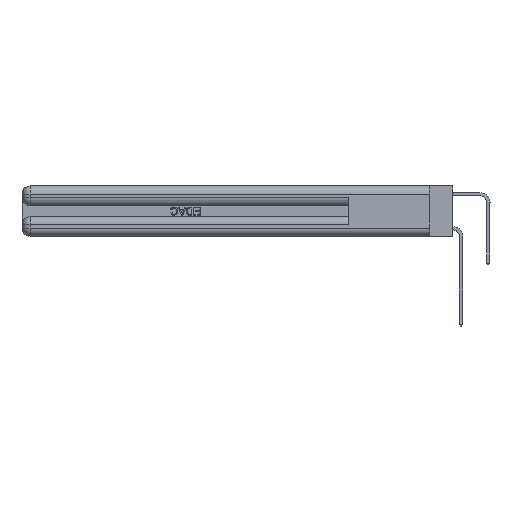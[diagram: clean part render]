
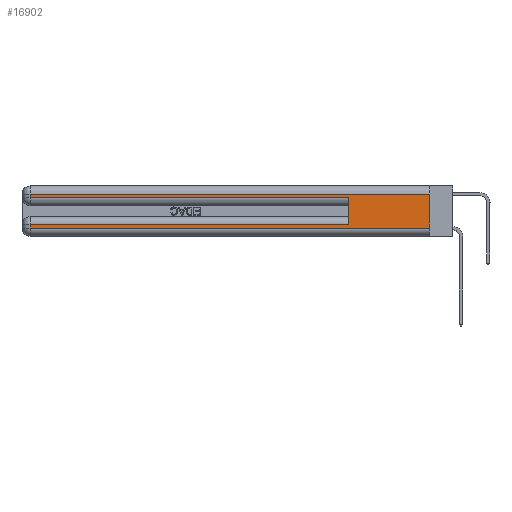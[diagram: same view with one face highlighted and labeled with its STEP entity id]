
A CAD part, left-side view. The second image highlights one B-rep face of the part: STEP entity #16902.
In plain terms, the highlighted planar face has unit normal (-1, 0, 0).
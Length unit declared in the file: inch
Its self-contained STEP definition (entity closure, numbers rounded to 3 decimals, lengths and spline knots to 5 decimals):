
#387 = ORIENTED_EDGE ( 'NONE', *, *, #13676, .T. ) ;
#787 = ORIENTED_EDGE ( 'NONE', *, *, #15017, .F. ) ;
#1704 = ORIENTED_EDGE ( 'NONE', *, *, #35412, .T. ) ;
#2054 = VERTEX_POINT ( 'NONE', #36527 ) ;
#2170 = LINE ( 'NONE', #22982, #8483 ) ;
#2703 = VERTEX_POINT ( 'NONE', #21536 ) ;
#3067 = VECTOR ( 'NONE', #14530, 39.37008 ) ;
#3115 = ORIENTED_EDGE ( 'NONE', *, *, #11278, .T. ) ;
#4183 = CARTESIAN_POINT ( 'NONE',  ( 0., 0., 0.31 ) ) ;
#4796 = FACE_OUTER_BOUND ( 'NONE', #35526, .T. ) ;
#5351 = DIRECTION ( 'NONE',  ( 0., -1., 0. ) ) ;
#6927 = CARTESIAN_POINT ( 'NONE',  ( 0., 0., 0.31 ) ) ;
#8483 = VECTOR ( 'NONE', #12206, 39.37008 ) ;
#8495 = VERTEX_POINT ( 'NONE', #32605 ) ;
#8623 = DIRECTION ( 'NONE',  ( 0., 0., -1. ) ) ;
#8759 = VECTOR ( 'NONE', #23881, 39.37008 ) ;
#9619 = VECTOR ( 'NONE', #36544, 39.37008 ) ;
#10523 = VECTOR ( 'NONE', #14014, 39.37008 ) ;
#11159 = CARTESIAN_POINT ( 'NONE',  ( 0., 0., 0.085 ) ) ;
#11278 = EDGE_CURVE ( 'NONE', #8495, #20273, #33850, .T. ) ;
#12206 = DIRECTION ( 'NONE',  ( 0., 0., -1. ) ) ;
#12782 = CARTESIAN_POINT ( 'NONE',  ( 0., 2.94, 0.37 ) ) ;
#13591 = LINE ( 'NONE', #28121, #9619 ) ;
#13676 = EDGE_CURVE ( 'NONE', #36613, #35907, #14814, .T. ) ;
#14014 = DIRECTION ( 'NONE',  ( 0., 1., 0. ) ) ;
#14047 = ORIENTED_EDGE ( 'NONE', *, *, #31770, .T. ) ;
#14053 = CARTESIAN_POINT ( 'NONE',  ( 0., 0.6, 0.285 ) ) ;
#14530 = DIRECTION ( 'NONE',  ( 0., 0., 1. ) ) ;
#14814 = LINE ( 'NONE', #6927, #22422 ) ;
#15017 = EDGE_CURVE ( 'NONE', #8495, #18442, #30423, .T. ) ;
#15422 = ORIENTED_EDGE ( 'NONE', *, *, #18229, .T. ) ;
#16496 = ORIENTED_EDGE ( 'NONE', *, *, #29160, .T. ) ;
#16902 = ADVANCED_FACE ( 'NONE', ( #4796 ), #19937, .F. ) ;
#17740 = CARTESIAN_POINT ( 'NONE',  ( 0., 2.94, 0.06 ) ) ;
#18229 = EDGE_CURVE ( 'NONE', #35907, #2054, #26160, .T. ) ;
#18442 = VERTEX_POINT ( 'NONE', #14053 ) ;
#18483 = LINE ( 'NONE', #20409, #31954 ) ;
#19937 = PLANE ( 'NONE',  #24099 ) ;
#20106 = EDGE_CURVE ( 'NONE', #36613, #2703, #18483, .T. ) ;
#20273 = VERTEX_POINT ( 'NONE', #30600 ) ;
#20409 = CARTESIAN_POINT ( 'NONE',  ( 0., 0., 0.37 ) ) ;
#21045 = ORIENTED_EDGE ( 'NONE', *, *, #20106, .F. ) ;
#21076 = CARTESIAN_POINT ( 'NONE',  ( 0., 2.94, 0.31 ) ) ;
#21536 = CARTESIAN_POINT ( 'NONE',  ( 0., 0., 0.06 ) ) ;
#22422 = VECTOR ( 'NONE', #33861, 39.37008 ) ;
#22568 = CARTESIAN_POINT ( 'NONE',  ( 0., 0., 0.37 ) ) ;
#22702 = DIRECTION ( 'NONE',  ( 1., 0., 0. ) ) ;
#22982 = CARTESIAN_POINT ( 'NONE',  ( 0., 2.94, 0.37 ) ) ;
#23633 = CARTESIAN_POINT ( 'NONE',  ( 0., 0.6, 0.145 ) ) ;
#23881 = DIRECTION ( 'NONE',  ( 0., 0., -1. ) ) ;
#24099 = AXIS2_PLACEMENT_3D ( 'NONE', #22568, #22702, #8623 ) ;
#25918 = VERTEX_POINT ( 'NONE', #17740 ) ;
#26160 = LINE ( 'NONE', #12782, #8759 ) ;
#28121 = CARTESIAN_POINT ( 'NONE',  ( 0., 0., 0.06 ) ) ;
#28499 = CARTESIAN_POINT ( 'NONE',  ( 0., 0., 0.285 ) ) ;
#29160 = EDGE_CURVE ( 'NONE', #25918, #2703, #13591, .T. ) ;
#30229 = LINE ( 'NONE', #28499, #36982 ) ;
#30423 = LINE ( 'NONE', #23633, #3067 ) ;
#30600 = CARTESIAN_POINT ( 'NONE',  ( 0., 2.94, 0.085 ) ) ;
#31770 = EDGE_CURVE ( 'NONE', #2054, #18442, #30229, .T. ) ;
#31954 = VECTOR ( 'NONE', #34906, 39.37008 ) ;
#32605 = CARTESIAN_POINT ( 'NONE',  ( 0., 0.6, 0.085 ) ) ;
#33850 = LINE ( 'NONE', #11159, #10523 ) ;
#33861 = DIRECTION ( 'NONE',  ( 0., 1., 0. ) ) ;
#34906 = DIRECTION ( 'NONE',  ( 0., 0., -1. ) ) ;
#35412 = EDGE_CURVE ( 'NONE', #20273, #25918, #2170, .T. ) ;
#35526 = EDGE_LOOP ( 'NONE', ( #21045, #387, #15422, #14047, #787, #3115, #1704, #16496 ) ) ;
#35907 = VERTEX_POINT ( 'NONE', #21076 ) ;
#36527 = CARTESIAN_POINT ( 'NONE',  ( 0., 2.94, 0.285 ) ) ;
#36544 = DIRECTION ( 'NONE',  ( 0., -1., 0. ) ) ;
#36613 = VERTEX_POINT ( 'NONE', #4183 ) ;
#36982 = VECTOR ( 'NONE', #5351, 39.37008 ) ;
